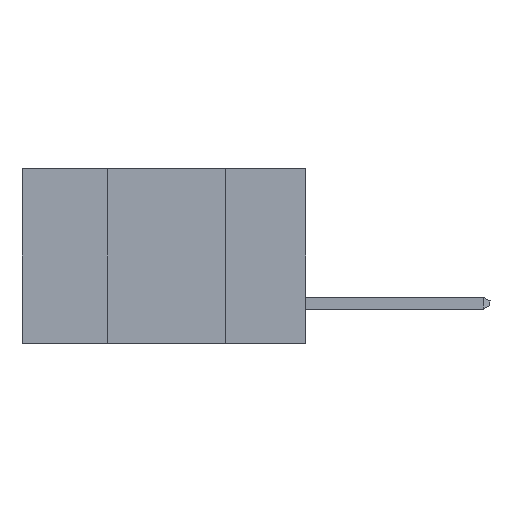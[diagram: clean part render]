
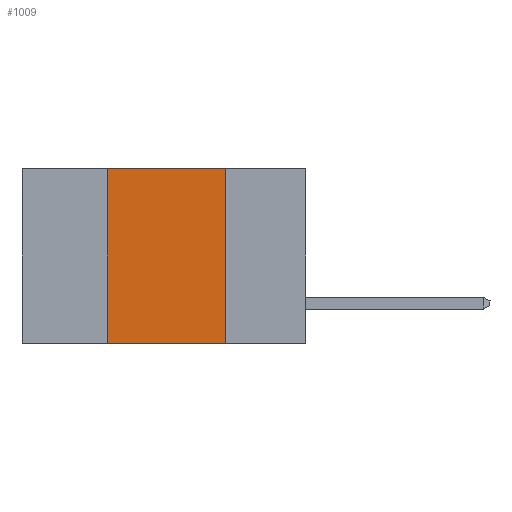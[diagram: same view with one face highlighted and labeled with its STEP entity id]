
A CAD part, left-side view. The second image highlights one B-rep face of the part: STEP entity #1009.
In plain terms, the highlighted planar face has unit normal (-1, 0, 0).
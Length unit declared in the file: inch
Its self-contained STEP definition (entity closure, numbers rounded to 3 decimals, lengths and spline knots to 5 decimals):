
#599 = DIRECTION ( 'NONE',  ( 0., 0., 1. ) ) ;
#604 = VERTEX_POINT ( 'NONE', #6690 ) ;
#621 = ORIENTED_EDGE ( 'NONE', *, *, #8926, .F. ) ;
#1009 = ADVANCED_FACE ( 'NONE', ( #4347 ), #2967, .F. ) ;
#2451 = VECTOR ( 'NONE', #7846, 39.37008 ) ;
#2706 = DIRECTION ( 'NONE',  ( 0., -1., 0. ) ) ;
#2842 = AXIS2_PLACEMENT_3D ( 'NONE', #6346, #4214, #4898 ) ;
#2967 = PLANE ( 'NONE',  #2842 ) ;
#3140 = EDGE_CURVE ( 'NONE', #604, #3641, #6304, .T. ) ;
#3641 = VERTEX_POINT ( 'NONE', #5978 ) ;
#3734 = ORIENTED_EDGE ( 'NONE', *, *, #3140, .T. ) ;
#4085 = LINE ( 'NONE', #7626, #4191 ) ;
#4191 = VECTOR ( 'NONE', #8973, 39.37008 ) ;
#4214 = DIRECTION ( 'NONE',  ( 1., 0., 0. ) ) ;
#4347 = FACE_OUTER_BOUND ( 'NONE', #7737, .T. ) ;
#4661 = CARTESIAN_POINT ( 'NONE',  ( 0., 0.17, 0. ) ) ;
#4897 = CARTESIAN_POINT ( 'NONE',  ( 0., 0.6, 0. ) ) ;
#4898 = DIRECTION ( 'NONE',  ( 0., 0., -1. ) ) ;
#4987 = LINE ( 'NONE', #4897, #6010 ) ;
#5083 = CARTESIAN_POINT ( 'NONE',  ( 0., 0.6, -0.37 ) ) ;
#5478 = CARTESIAN_POINT ( 'NONE',  ( 0., 0.42, 0. ) ) ;
#5615 = LINE ( 'NONE', #7608, #6715 ) ;
#5978 = CARTESIAN_POINT ( 'NONE',  ( 0., 0.17, -0.37 ) ) ;
#6010 = VECTOR ( 'NONE', #2706, 39.37008 ) ;
#6304 = LINE ( 'NONE', #5083, #2451 ) ;
#6346 = CARTESIAN_POINT ( 'NONE',  ( 0., 0.6, 0. ) ) ;
#6669 = ORIENTED_EDGE ( 'NONE', *, *, #8119, .F. ) ;
#6690 = CARTESIAN_POINT ( 'NONE',  ( 0., 0.42, -0.37 ) ) ;
#6715 = VECTOR ( 'NONE', #599, 39.37008 ) ;
#6778 = VERTEX_POINT ( 'NONE', #4661 ) ;
#6934 = VERTEX_POINT ( 'NONE', #5478 ) ;
#7406 = ORIENTED_EDGE ( 'NONE', *, *, #7831, .F. ) ;
#7608 = CARTESIAN_POINT ( 'NONE',  ( 0., 0.42, -0.37 ) ) ;
#7626 = CARTESIAN_POINT ( 'NONE',  ( 0., 0.17, -0.37 ) ) ;
#7737 = EDGE_LOOP ( 'NONE', ( #621, #7406, #6669, #3734 ) ) ;
#7831 = EDGE_CURVE ( 'NONE', #6934, #6778, #4987, .T. ) ;
#7846 = DIRECTION ( 'NONE',  ( 0., -1., 0. ) ) ;
#8119 = EDGE_CURVE ( 'NONE', #604, #6934, #5615, .T. ) ;
#8926 = EDGE_CURVE ( 'NONE', #6778, #3641, #4085, .T. ) ;
#8973 = DIRECTION ( 'NONE',  ( 0., 0., -1. ) ) ;
